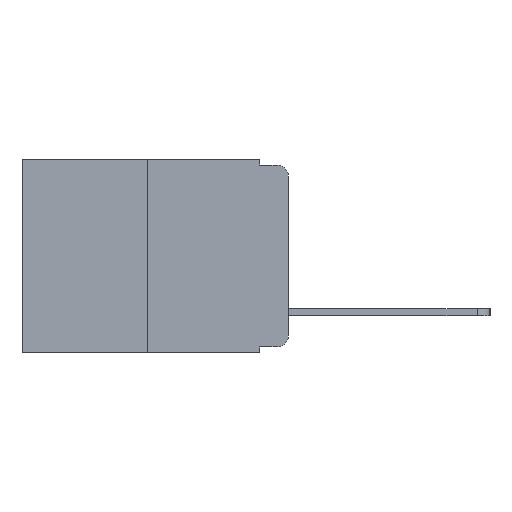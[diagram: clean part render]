
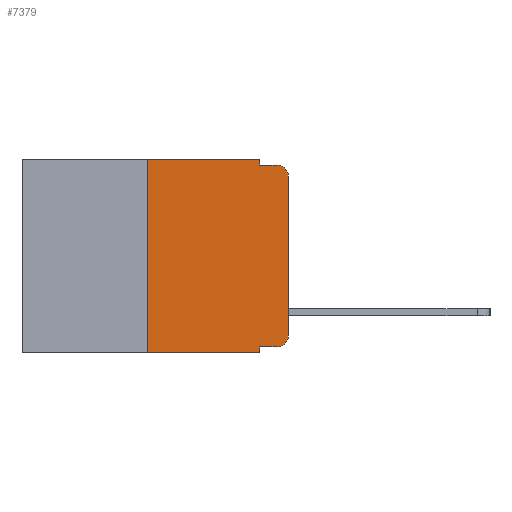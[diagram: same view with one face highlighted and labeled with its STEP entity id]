
A CAD part, left-side view. The second image highlights one B-rep face of the part: STEP entity #7379.
In plain terms, the highlighted planar face has unit normal (-1, 0, 0).
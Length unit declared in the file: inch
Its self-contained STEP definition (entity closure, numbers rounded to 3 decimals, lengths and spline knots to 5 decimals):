
#46 = ORIENTED_EDGE ( 'NONE', *, *, #11514, .T. ) ;
#300 = LINE ( 'NONE', #4564, #5460 ) ;
#439 = AXIS2_PLACEMENT_3D ( 'NONE', #5225, #11090, #6140 ) ;
#457 = EDGE_CURVE ( 'NONE', #7153, #11588, #7533, .T. ) ;
#772 = DIRECTION ( 'NONE',  ( 0., 0., -1. ) ) ;
#797 = DIRECTION ( 'NONE',  ( -1., 0., 0. ) ) ;
#893 = VECTOR ( 'NONE', #10291, 39.37008 ) ;
#1110 = DIRECTION ( 'NONE',  ( 0., 0., -1. ) ) ;
#1151 = LINE ( 'NONE', #9066, #6434 ) ;
#1160 = CARTESIAN_POINT ( 'NONE',  ( 0., 0.051, 0. ) ) ;
#1456 = VERTEX_POINT ( 'NONE', #6901 ) ;
#1605 = VECTOR ( 'NONE', #1110, 39.37008 ) ;
#2113 = EDGE_CURVE ( 'NONE', #5032, #10117, #6585, .T. ) ;
#2245 = ORIENTED_EDGE ( 'NONE', *, *, #9113, .F. ) ;
#2643 = ORIENTED_EDGE ( 'NONE', *, *, #10744, .T. ) ;
#2767 = VERTEX_POINT ( 'NONE', #4667 ) ;
#2775 = EDGE_CURVE ( 'NONE', #2767, #10117, #1151, .T. ) ;
#2853 = CARTESIAN_POINT ( 'NONE',  ( 0., 0., 0. ) ) ;
#3081 = DIRECTION ( 'NONE',  ( 1., 0., 0. ) ) ;
#3702 = EDGE_CURVE ( 'NONE', #11588, #4194, #5898, .T. ) ;
#3783 = CARTESIAN_POINT ( 'NONE',  ( 0., 0.051, -0.343 ) ) ;
#3894 = CARTESIAN_POINT ( 'NONE',  ( 0., 0.051, 0. ) ) ;
#3973 = CARTESIAN_POINT ( 'NONE',  ( 0., 0.051, 0. ) ) ;
#4069 = CIRCLE ( 'NONE', #439, 0.02 ) ;
#4194 = VERTEX_POINT ( 'NONE', #4640 ) ;
#4232 = VECTOR ( 'NONE', #6190, 39.37008 ) ;
#4564 = CARTESIAN_POINT ( 'NONE',  ( 0., 0.473, 0. ) ) ;
#4640 = CARTESIAN_POINT ( 'NONE',  ( 0., 0.02, -0.01 ) ) ;
#4667 = CARTESIAN_POINT ( 'NONE',  ( 0., 0.25, -0.343 ) ) ;
#5032 = VERTEX_POINT ( 'NONE', #8099 ) ;
#5225 = CARTESIAN_POINT ( 'NONE',  ( 0., 0.02, -0.313 ) ) ;
#5236 = VECTOR ( 'NONE', #9807, 39.37008 ) ;
#5416 = EDGE_CURVE ( 'NONE', #2767, #9091, #7929, .T. ) ;
#5460 = VECTOR ( 'NONE', #11361, 39.37008 ) ;
#5596 = VECTOR ( 'NONE', #9162, 39.37008 ) ;
#5738 = VERTEX_POINT ( 'NONE', #1160 ) ;
#5759 = VECTOR ( 'NONE', #8759, 39.37008 ) ;
#5848 = ORIENTED_EDGE ( 'NONE', *, *, #5416, .F. ) ;
#5898 = CIRCLE ( 'NONE', #9747, 0.02 ) ;
#6140 = DIRECTION ( 'NONE',  ( 0., 0., -1. ) ) ;
#6190 = DIRECTION ( 'NONE',  ( 0., -1., 0. ) ) ;
#6369 = CARTESIAN_POINT ( 'NONE',  ( 0., 0.25, 0. ) ) ;
#6434 = VECTOR ( 'NONE', #10000, 39.37008 ) ;
#6585 = LINE ( 'NONE', #3973, #1605 ) ;
#6765 = PLANE ( 'NONE',  #10286 ) ;
#6901 = CARTESIAN_POINT ( 'NONE',  ( 0., 0.051, -0.01 ) ) ;
#6965 = CARTESIAN_POINT ( 'NONE',  ( 0., 0., -0.313 ) ) ;
#7153 = VERTEX_POINT ( 'NONE', #6965 ) ;
#7379 = ADVANCED_FACE ( 'NONE', ( #7905 ), #6765, .F. ) ;
#7514 = ORIENTED_EDGE ( 'NONE', *, *, #3702, .T. ) ;
#7533 = LINE ( 'NONE', #2853, #5236 ) ;
#7788 = ORIENTED_EDGE ( 'NONE', *, *, #9048, .F. ) ;
#7856 = LINE ( 'NONE', #3894, #5596 ) ;
#7905 = FACE_OUTER_BOUND ( 'NONE', #8883, .T. ) ;
#7929 = LINE ( 'NONE', #8635, #893 ) ;
#7953 = ORIENTED_EDGE ( 'NONE', *, *, #2775, .T. ) ;
#7974 = CARTESIAN_POINT ( 'NONE',  ( 0., 0.051, -0.01 ) ) ;
#7988 = LINE ( 'NONE', #7974, #5759 ) ;
#8047 = CARTESIAN_POINT ( 'NONE',  ( 0., 0.02, -0.333 ) ) ;
#8099 = CARTESIAN_POINT ( 'NONE',  ( 0., 0.051, -0.333 ) ) ;
#8445 = CARTESIAN_POINT ( 'NONE',  ( 0., 0.473, 0. ) ) ;
#8635 = CARTESIAN_POINT ( 'NONE',  ( 0., 0.25, 0. ) ) ;
#8759 = DIRECTION ( 'NONE',  ( 0., -1., 0. ) ) ;
#8883 = EDGE_LOOP ( 'NONE', ( #11458, #7514, #7788, #9031, #2245, #5848, #7953, #9076, #2643, #46 ) ) ;
#9031 = ORIENTED_EDGE ( 'NONE', *, *, #9371, .F. ) ;
#9048 = EDGE_CURVE ( 'NONE', #1456, #4194, #7988, .T. ) ;
#9066 = CARTESIAN_POINT ( 'NONE',  ( 0., 0.473, -0.343 ) ) ;
#9076 = ORIENTED_EDGE ( 'NONE', *, *, #2113, .F. ) ;
#9091 = VERTEX_POINT ( 'NONE', #6369 ) ;
#9100 = VERTEX_POINT ( 'NONE', #8047 ) ;
#9113 = EDGE_CURVE ( 'NONE', #9091, #5738, #300, .T. ) ;
#9162 = DIRECTION ( 'NONE',  ( 0., 0., -1. ) ) ;
#9268 = DIRECTION ( 'NONE',  ( 0., 0., -1. ) ) ;
#9371 = EDGE_CURVE ( 'NONE', #5738, #1456, #7856, .T. ) ;
#9747 = AXIS2_PLACEMENT_3D ( 'NONE', #11235, #797, #772 ) ;
#9807 = DIRECTION ( 'NONE',  ( 0., 0., 1. ) ) ;
#10000 = DIRECTION ( 'NONE',  ( 0., -1., 0. ) ) ;
#10117 = VERTEX_POINT ( 'NONE', #3783 ) ;
#10286 = AXIS2_PLACEMENT_3D ( 'NONE', #8445, #3081, #9268 ) ;
#10291 = DIRECTION ( 'NONE',  ( 0., 0., 1. ) ) ;
#10338 = CARTESIAN_POINT ( 'NONE',  ( 0., 0., -0.03 ) ) ;
#10744 = EDGE_CURVE ( 'NONE', #5032, #9100, #11044, .T. ) ;
#11044 = LINE ( 'NONE', #11141, #4232 ) ;
#11090 = DIRECTION ( 'NONE',  ( -1., 0., 0. ) ) ;
#11141 = CARTESIAN_POINT ( 'NONE',  ( 0., 0.051, -0.333 ) ) ;
#11235 = CARTESIAN_POINT ( 'NONE',  ( 0., 0.02, -0.03 ) ) ;
#11361 = DIRECTION ( 'NONE',  ( 0., -1., 0. ) ) ;
#11458 = ORIENTED_EDGE ( 'NONE', *, *, #457, .T. ) ;
#11514 = EDGE_CURVE ( 'NONE', #9100, #7153, #4069, .T. ) ;
#11588 = VERTEX_POINT ( 'NONE', #10338 ) ;
